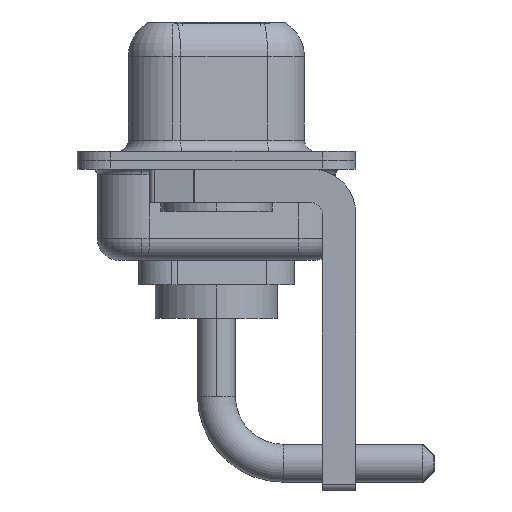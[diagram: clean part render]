
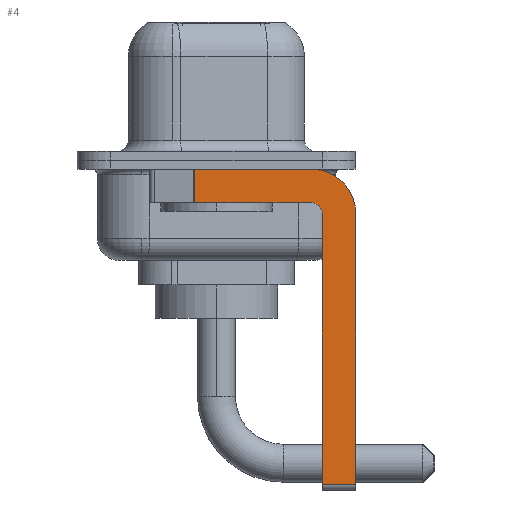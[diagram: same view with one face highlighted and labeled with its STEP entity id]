
A CAD part, left-side view. The second image highlights one B-rep face of the part: STEP entity #4.
In plain terms, the highlighted planar face has unit normal (-1, 0, 0).
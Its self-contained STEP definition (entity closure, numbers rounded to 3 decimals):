
#4 = ADVANCED_FACE ( 'NONE', ( #8166 ), #11323, .F. ) ;
#33 = AXIS2_PLACEMENT_3D ( 'NONE', #7006, #12502, #11467 ) ;
#36 = CARTESIAN_POINT ( 'NONE',  ( -2.9, -4.25, -2.4 ) ) ;
#139 = VERTEX_POINT ( 'NONE', #7295 ) ;
#317 = CARTESIAN_POINT ( 'NONE',  ( -2.9, -4.75, -14.8 ) ) ;
#450 = DIRECTION ( 'NONE',  ( 0., -1., 0. ) ) ;
#527 = CARTESIAN_POINT ( 'NONE',  ( -2.9, 3., -0.4 ) ) ;
#554 = ORIENTED_EDGE ( 'NONE', *, *, #4170, .F. ) ;
#638 = CARTESIAN_POINT ( 'NONE',  ( -2.9, -4.75, -2.4 ) ) ;
#1345 = DIRECTION ( 'NONE',  ( 0., 0., 1. ) ) ;
#2171 = DIRECTION ( 'NONE',  ( 1., 0., 0. ) ) ;
#2377 = DIRECTION ( 'NONE',  ( 0., 0., -1. ) ) ;
#2418 = EDGE_CURVE ( 'NONE', #13322, #6068, #4336, .T. ) ;
#2421 = EDGE_LOOP ( 'NONE', ( #2429, #4890, #2719, #11941, #554, #14339, #5593, #12430 ) ) ;
#2429 = ORIENTED_EDGE ( 'NONE', *, *, #5941, .F. ) ;
#2719 = ORIENTED_EDGE ( 'NONE', *, *, #14157, .F. ) ;
#3618 = AXIS2_PLACEMENT_3D ( 'NONE', #12476, #11367, #12628 ) ;
#3810 = VECTOR ( 'NONE', #6327, 1000. ) ;
#3935 = VERTEX_POINT ( 'NONE', #9873 ) ;
#4170 = EDGE_CURVE ( 'NONE', #10219, #13322, #13622, .T. ) ;
#4193 = LINE ( 'NONE', #9716, #10694 ) ;
#4309 = CARTESIAN_POINT ( 'NONE',  ( -2.9, 0.978, -1.9 ) ) ;
#4336 = CIRCLE ( 'NONE', #3618, 0.5 ) ;
#4399 = VECTOR ( 'NONE', #450, 1000. ) ;
#4714 = CARTESIAN_POINT ( 'NONE',  ( -2.9, -4.75, -14.55 ) ) ;
#4880 = CARTESIAN_POINT ( 'NONE',  ( -2.9, -6.25, -2.4 ) ) ;
#4890 = ORIENTED_EDGE ( 'NONE', *, *, #10704, .T. ) ;
#4908 = VERTEX_POINT ( 'NONE', #6956 ) ;
#5593 = ORIENTED_EDGE ( 'NONE', *, *, #8516, .F. ) ;
#5941 = EDGE_CURVE ( 'NONE', #3935, #139, #7356, .T. ) ;
#6068 = VERTEX_POINT ( 'NONE', #6618 ) ;
#6327 = DIRECTION ( 'NONE',  ( 0., -1., 0. ) ) ;
#6538 = EDGE_CURVE ( 'NONE', #139, #9835, #6674, .T. ) ;
#6618 = CARTESIAN_POINT ( 'NONE',  ( -2.9, -4.25, -1.9 ) ) ;
#6674 = CIRCLE ( 'NONE', #10893, 2. ) ;
#6956 = CARTESIAN_POINT ( 'NONE',  ( -2.9, -6.25, -14.55 ) ) ;
#7006 = CARTESIAN_POINT ( 'NONE',  ( -2.9, -4.25, -2.4 ) ) ;
#7295 = CARTESIAN_POINT ( 'NONE',  ( -2.9, -4.25, -0.4 ) ) ;
#7356 = LINE ( 'NONE', #527, #3810 ) ;
#8166 = FACE_OUTER_BOUND ( 'NONE', #2421, .T. ) ;
#8516 = EDGE_CURVE ( 'NONE', #9835, #4908, #4193, .T. ) ;
#9390 = LINE ( 'NONE', #13473, #11915 ) ;
#9716 = CARTESIAN_POINT ( 'NONE',  ( -2.9, -6.25, -2.4 ) ) ;
#9788 = DIRECTION ( 'NONE',  ( 0., 0., -1. ) ) ;
#9835 = VERTEX_POINT ( 'NONE', #4880 ) ;
#9873 = CARTESIAN_POINT ( 'NONE',  ( -2.9, 0.978, -0.4 ) ) ;
#10075 = DIRECTION ( 'NONE',  ( 0., 0., -1. ) ) ;
#10219 = VERTEX_POINT ( 'NONE', #4714 ) ;
#10500 = CARTESIAN_POINT ( 'NONE',  ( -2.9, -4.25, -14.55 ) ) ;
#10694 = VECTOR ( 'NONE', #9788, 1000. ) ;
#10704 = EDGE_CURVE ( 'NONE', #3935, #14228, #9390, .T. ) ;
#10893 = AXIS2_PLACEMENT_3D ( 'NONE', #36, #2171, #2377 ) ;
#11323 = PLANE ( 'NONE',  #33 ) ;
#11367 = DIRECTION ( 'NONE',  ( -1., 0., 0. ) ) ;
#11467 = DIRECTION ( 'NONE',  ( 0., 0., -1. ) ) ;
#11915 = VECTOR ( 'NONE', #10075, 1000. ) ;
#11941 = ORIENTED_EDGE ( 'NONE', *, *, #2418, .F. ) ;
#12269 = EDGE_CURVE ( 'NONE', #10219, #4908, #12712, .T. ) ;
#12271 = VECTOR ( 'NONE', #1345, 1000. ) ;
#12427 = CARTESIAN_POINT ( 'NONE',  ( -2.9, -4.25, -1.9 ) ) ;
#12430 = ORIENTED_EDGE ( 'NONE', *, *, #6538, .F. ) ;
#12476 = CARTESIAN_POINT ( 'NONE',  ( -2.9, -4.25, -2.4 ) ) ;
#12502 = DIRECTION ( 'NONE',  ( 1., 0., 0. ) ) ;
#12628 = DIRECTION ( 'NONE',  ( 0., 0., 1. ) ) ;
#12670 = VECTOR ( 'NONE', #13818, 1000. ) ;
#12712 = LINE ( 'NONE', #10500, #4399 ) ;
#12857 = LINE ( 'NONE', #12427, #12670 ) ;
#13322 = VERTEX_POINT ( 'NONE', #638 ) ;
#13473 = CARTESIAN_POINT ( 'NONE',  ( -2.9, 0.978, -1.9 ) ) ;
#13622 = LINE ( 'NONE', #317, #12271 ) ;
#13818 = DIRECTION ( 'NONE',  ( 0., 1., 0. ) ) ;
#14157 = EDGE_CURVE ( 'NONE', #6068, #14228, #12857, .T. ) ;
#14228 = VERTEX_POINT ( 'NONE', #4309 ) ;
#14339 = ORIENTED_EDGE ( 'NONE', *, *, #12269, .T. ) ;
